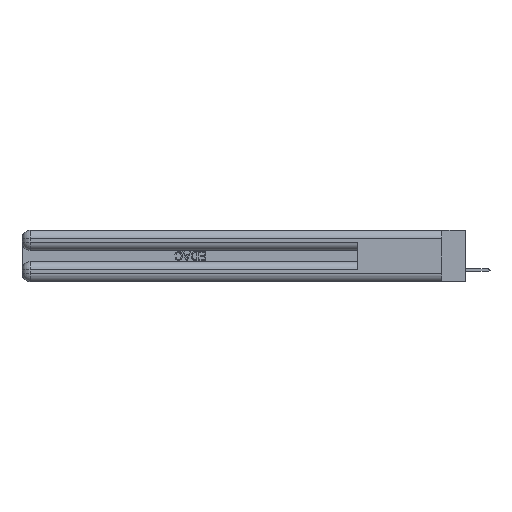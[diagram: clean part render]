
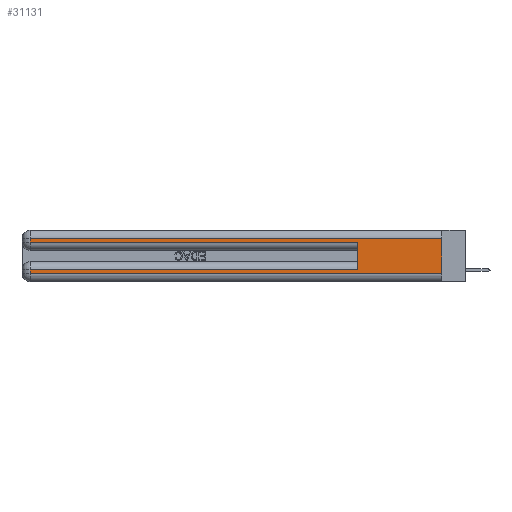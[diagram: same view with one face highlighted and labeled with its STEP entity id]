
A CAD part, left-side view. The second image highlights one B-rep face of the part: STEP entity #31131.
In plain terms, the highlighted planar face has unit normal (-1, 0, 0).
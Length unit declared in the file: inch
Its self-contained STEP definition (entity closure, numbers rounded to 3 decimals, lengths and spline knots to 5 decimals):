
#136 = LINE ( 'NONE', #13769, #29506 ) ;
#918 = LINE ( 'NONE', #17019, #2520 ) ;
#1577 = VERTEX_POINT ( 'NONE', #16263 ) ;
#1654 = LINE ( 'NONE', #19766, #26414 ) ;
#2259 = VERTEX_POINT ( 'NONE', #32399 ) ;
#2520 = VECTOR ( 'NONE', #9229, 39.37008 ) ;
#4602 = EDGE_CURVE ( 'NONE', #25722, #16430, #23683, .T. ) ;
#6659 = VECTOR ( 'NONE', #21464, 39.37008 ) ;
#7391 = EDGE_CURVE ( 'NONE', #2259, #1577, #1654, .T. ) ;
#7564 = ORIENTED_EDGE ( 'NONE', *, *, #7788, .T. ) ;
#7788 = EDGE_CURVE ( 'NONE', #33778, #1577, #23919, .T. ) ;
#7837 = ORIENTED_EDGE ( 'NONE', *, *, #24268, .T. ) ;
#7960 = ORIENTED_EDGE ( 'NONE', *, *, #18637, .T. ) ;
#8374 = PLANE ( 'NONE',  #31208 ) ;
#8547 = CARTESIAN_POINT ( 'NONE',  ( 0., 0., 0.06 ) ) ;
#9229 = DIRECTION ( 'NONE',  ( 0., 0., -1. ) ) ;
#9519 = EDGE_CURVE ( 'NONE', #31736, #30058, #918, .T. ) ;
#11943 = VERTEX_POINT ( 'NONE', #24174 ) ;
#12300 = DIRECTION ( 'NONE',  ( 0., 1., 0. ) ) ;
#12354 = VECTOR ( 'NONE', #26685, 39.37008 ) ;
#13458 = ORIENTED_EDGE ( 'NONE', *, *, #39772, .T. ) ;
#13769 = CARTESIAN_POINT ( 'NONE',  ( 0., 2.94, 0.37 ) ) ;
#14696 = CARTESIAN_POINT ( 'NONE',  ( 0., 2.94, 0.285 ) ) ;
#15632 = DIRECTION ( 'NONE',  ( 0., 0., 1. ) ) ;
#16263 = CARTESIAN_POINT ( 'NONE',  ( 0., 0., 0.06 ) ) ;
#16430 = VERTEX_POINT ( 'NONE', #33386 ) ;
#17019 = CARTESIAN_POINT ( 'NONE',  ( 0., 2.94, 0.37 ) ) ;
#17560 = DIRECTION ( 'NONE',  ( 0., 0., -1. ) ) ;
#18580 = CARTESIAN_POINT ( 'NONE',  ( 0., 0.6, 0.145 ) ) ;
#18637 = EDGE_CURVE ( 'NONE', #30058, #16430, #23377, .T. ) ;
#19193 = CARTESIAN_POINT ( 'NONE',  ( 0., 0., 0.085 ) ) ;
#19766 = CARTESIAN_POINT ( 'NONE',  ( 0., 0., 0.37 ) ) ;
#20054 = VECTOR ( 'NONE', #12300, 39.37008 ) ;
#20228 = CARTESIAN_POINT ( 'NONE',  ( 0., 0., 0.285 ) ) ;
#20266 = CARTESIAN_POINT ( 'NONE',  ( 0., 2.94, 0.31 ) ) ;
#21464 = DIRECTION ( 'NONE',  ( 0., -1., 0. ) ) ;
#21750 = LINE ( 'NONE', #23717, #39398 ) ;
#23377 = LINE ( 'NONE', #20228, #12354 ) ;
#23683 = LINE ( 'NONE', #18580, #36862 ) ;
#23717 = CARTESIAN_POINT ( 'NONE',  ( 0., 0., 0.31 ) ) ;
#23919 = LINE ( 'NONE', #8547, #6659 ) ;
#24174 = CARTESIAN_POINT ( 'NONE',  ( 0., 2.94, 0.085 ) ) ;
#24268 = EDGE_CURVE ( 'NONE', #25722, #11943, #38820, .T. ) ;
#24626 = DIRECTION ( 'NONE',  ( 0., 0., -1. ) ) ;
#25722 = VERTEX_POINT ( 'NONE', #34859 ) ;
#26414 = VECTOR ( 'NONE', #24626, 39.37008 ) ;
#26685 = DIRECTION ( 'NONE',  ( 0., -1., 0. ) ) ;
#26788 = DIRECTION ( 'NONE',  ( 0., 1., 0. ) ) ;
#27137 = CARTESIAN_POINT ( 'NONE',  ( 0., 0., 0.37 ) ) ;
#29506 = VECTOR ( 'NONE', #35972, 39.37008 ) ;
#29989 = EDGE_CURVE ( 'NONE', #2259, #31736, #21750, .T. ) ;
#30058 = VERTEX_POINT ( 'NONE', #14696 ) ;
#31131 = ADVANCED_FACE ( 'NONE', ( #36755 ), #8374, .F. ) ;
#31208 = AXIS2_PLACEMENT_3D ( 'NONE', #27137, #40653, #17560 ) ;
#31651 = ORIENTED_EDGE ( 'NONE', *, *, #4602, .F. ) ;
#31736 = VERTEX_POINT ( 'NONE', #20266 ) ;
#32399 = CARTESIAN_POINT ( 'NONE',  ( 0., 0., 0.31 ) ) ;
#32587 = EDGE_LOOP ( 'NONE', ( #38230, #35490, #41976, #7960, #31651, #7837, #13458, #7564 ) ) ;
#33386 = CARTESIAN_POINT ( 'NONE',  ( 0., 0.6, 0.285 ) ) ;
#33778 = VERTEX_POINT ( 'NONE', #38139 ) ;
#34859 = CARTESIAN_POINT ( 'NONE',  ( 0., 0.6, 0.085 ) ) ;
#35490 = ORIENTED_EDGE ( 'NONE', *, *, #29989, .T. ) ;
#35972 = DIRECTION ( 'NONE',  ( 0., 0., -1. ) ) ;
#36755 = FACE_OUTER_BOUND ( 'NONE', #32587, .T. ) ;
#36862 = VECTOR ( 'NONE', #15632, 39.37008 ) ;
#38139 = CARTESIAN_POINT ( 'NONE',  ( 0., 2.94, 0.06 ) ) ;
#38230 = ORIENTED_EDGE ( 'NONE', *, *, #7391, .F. ) ;
#38820 = LINE ( 'NONE', #19193, #20054 ) ;
#39398 = VECTOR ( 'NONE', #26788, 39.37008 ) ;
#39772 = EDGE_CURVE ( 'NONE', #11943, #33778, #136, .T. ) ;
#40653 = DIRECTION ( 'NONE',  ( 1., 0., 0. ) ) ;
#41976 = ORIENTED_EDGE ( 'NONE', *, *, #9519, .T. ) ;
